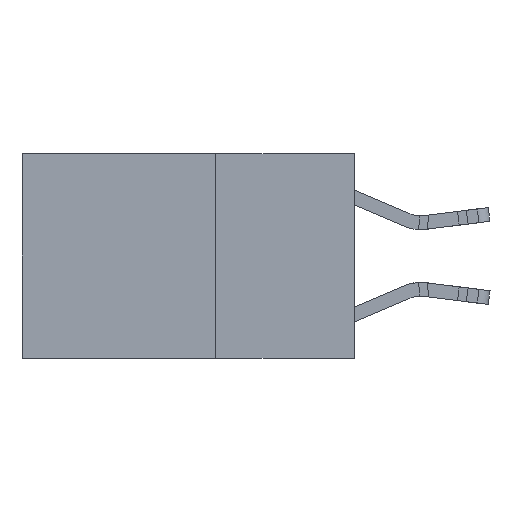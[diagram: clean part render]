
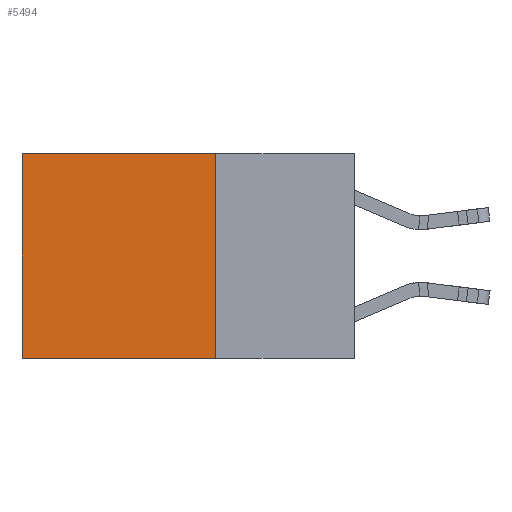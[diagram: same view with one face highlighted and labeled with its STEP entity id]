
A CAD part, left-side view. The second image highlights one B-rep face of the part: STEP entity #5494.
In plain terms, the highlighted planar face has unit normal (-1, 0, 0).
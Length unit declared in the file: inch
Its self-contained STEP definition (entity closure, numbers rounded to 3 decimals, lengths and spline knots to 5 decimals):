
#490 = EDGE_CURVE ( 'NONE', #16911, #23710, #27730, .T. ) ;
#2891 = CARTESIAN_POINT ( 'NONE',  ( 0.2625, 0.25, 0. ) ) ;
#3128 = AXIS2_PLACEMENT_3D ( 'NONE', #22061, #8717, #24269 ) ;
#3349 = EDGE_CURVE ( 'NONE', #23710, #12056, #27899, .T. ) ;
#3658 = EDGE_LOOP ( 'NONE', ( #14482, #15180, #9934, #21801 ) ) ;
#3724 = CARTESIAN_POINT ( 'NONE',  ( 0.2625, 0.25, -0.37 ) ) ;
#4397 = LINE ( 'NONE', #19541, #15540 ) ;
#5494 = ADVANCED_FACE ( 'NONE', ( #23149 ), #6514, .F. ) ;
#6514 = PLANE ( 'NONE',  #3128 ) ;
#7092 = CARTESIAN_POINT ( 'NONE',  ( 0.2625, 0.25, -0.37 ) ) ;
#8717 = DIRECTION ( 'NONE',  ( 1., 0., 0. ) ) ;
#9287 = DIRECTION ( 'NONE',  ( 0., 1., 0. ) ) ;
#9934 = ORIENTED_EDGE ( 'NONE', *, *, #490, .F. ) ;
#10397 = EDGE_CURVE ( 'NONE', #16911, #12322, #17735, .T. ) ;
#12056 = VERTEX_POINT ( 'NONE', #12554 ) ;
#12322 = VERTEX_POINT ( 'NONE', #15873 ) ;
#12554 = CARTESIAN_POINT ( 'NONE',  ( 0.2625, 0.6, -0.37 ) ) ;
#14007 = DIRECTION ( 'NONE',  ( 0., 1., 0. ) ) ;
#14241 = CARTESIAN_POINT ( 'NONE',  ( 0.2625, 0.25, 0. ) ) ;
#14482 = ORIENTED_EDGE ( 'NONE', *, *, #23067, .T. ) ;
#15180 = ORIENTED_EDGE ( 'NONE', *, *, #3349, .F. ) ;
#15540 = VECTOR ( 'NONE', #21783, 39.37008 ) ;
#15873 = CARTESIAN_POINT ( 'NONE',  ( 0.2625, 0.6, 0. ) ) ;
#16911 = VERTEX_POINT ( 'NONE', #14241 ) ;
#17735 = LINE ( 'NONE', #2891, #28686 ) ;
#19362 = DIRECTION ( 'NONE',  ( 0., 0., -1. ) ) ;
#19541 = CARTESIAN_POINT ( 'NONE',  ( 0.2625, 0.6, 0. ) ) ;
#21429 = VECTOR ( 'NONE', #9287, 39.37008 ) ;
#21783 = DIRECTION ( 'NONE',  ( 0., 0., -1. ) ) ;
#21801 = ORIENTED_EDGE ( 'NONE', *, *, #10397, .T. ) ;
#22061 = CARTESIAN_POINT ( 'NONE',  ( 0.2625, 0.25, 0. ) ) ;
#22642 = VECTOR ( 'NONE', #19362, 39.37008 ) ;
#23067 = EDGE_CURVE ( 'NONE', #12322, #12056, #4397, .T. ) ;
#23149 = FACE_OUTER_BOUND ( 'NONE', #3658, .T. ) ;
#23526 = CARTESIAN_POINT ( 'NONE',  ( 0.2625, 0.25, 0. ) ) ;
#23710 = VERTEX_POINT ( 'NONE', #3724 ) ;
#24269 = DIRECTION ( 'NONE',  ( 0., 0., -1. ) ) ;
#27730 = LINE ( 'NONE', #23526, #22642 ) ;
#27899 = LINE ( 'NONE', #7092, #21429 ) ;
#28686 = VECTOR ( 'NONE', #14007, 39.37008 ) ;
